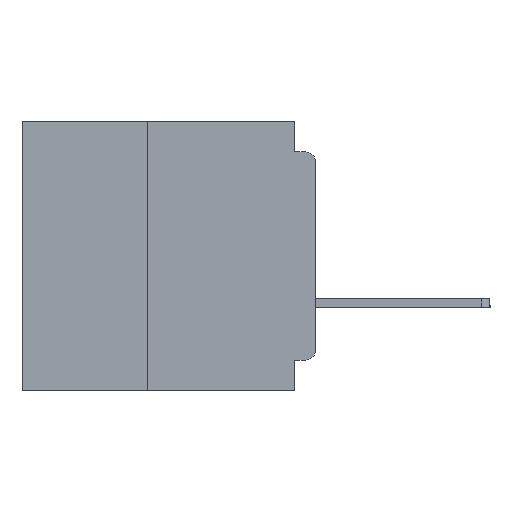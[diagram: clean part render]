
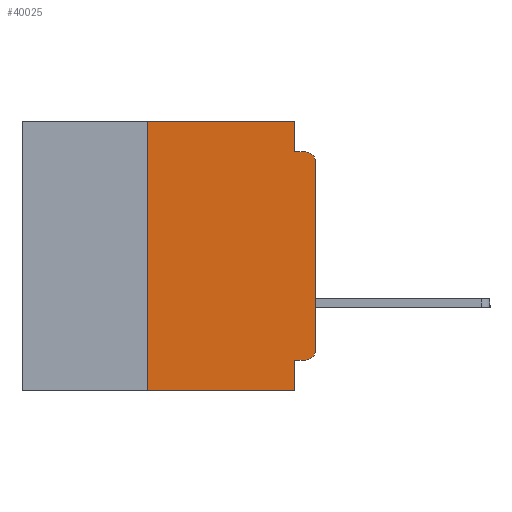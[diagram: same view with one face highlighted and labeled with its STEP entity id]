
A CAD part, left-side view. The second image highlights one B-rep face of the part: STEP entity #40025.
In plain terms, the highlighted planar face has unit normal (-1, 0, 0).
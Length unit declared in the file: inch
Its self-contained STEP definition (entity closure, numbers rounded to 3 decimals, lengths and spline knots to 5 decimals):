
#486 = LINE ( 'NONE', #40335, #39804 ) ;
#508 = VERTEX_POINT ( 'NONE', #45485 ) ;
#637 = LINE ( 'NONE', #27863, #26991 ) ;
#2961 = LINE ( 'NONE', #26568, #41119 ) ;
#3345 = LINE ( 'NONE', #22863, #11798 ) ;
#3546 = VERTEX_POINT ( 'NONE', #5297 ) ;
#5059 = CARTESIAN_POINT ( 'NONE',  ( 0., 0.031, -0.4 ) ) ;
#5124 = DIRECTION ( 'NONE',  ( 0., 1., 0. ) ) ;
#5297 = CARTESIAN_POINT ( 'NONE',  ( 0., 0.25, -0.4 ) ) ;
#5429 = DIRECTION ( 'NONE',  ( 0., 0., 1. ) ) ;
#5456 = CARTESIAN_POINT ( 'NONE',  ( 0., 0., -0.34 ) ) ;
#5501 = CARTESIAN_POINT ( 'NONE',  ( 0., 0.031, -0.4 ) ) ;
#5976 = VERTEX_POINT ( 'NONE', #9801 ) ;
#6390 = VERTEX_POINT ( 'NONE', #5501 ) ;
#8047 = VECTOR ( 'NONE', #38232, 39.37008 ) ;
#8141 = AXIS2_PLACEMENT_3D ( 'NONE', #34660, #13197, #38264 ) ;
#8829 = CARTESIAN_POINT ( 'NONE',  ( 0., 0.031, -0.045 ) ) ;
#8914 = CARTESIAN_POINT ( 'NONE',  ( 0., 0.25, -0.4 ) ) ;
#9580 = ORIENTED_EDGE ( 'NONE', *, *, #44940, .F. ) ;
#9801 = CARTESIAN_POINT ( 'NONE',  ( 0., 0., -0.06 ) ) ;
#10023 = DIRECTION ( 'NONE',  ( 0., -1., 0. ) ) ;
#10333 = LINE ( 'NONE', #45315, #29391 ) ;
#10429 = VERTEX_POINT ( 'NONE', #28794 ) ;
#10706 = CARTESIAN_POINT ( 'NONE',  ( 0., 0.031, 0. ) ) ;
#11145 = VERTEX_POINT ( 'NONE', #8829 ) ;
#11545 = VECTOR ( 'NONE', #13118, 39.37008 ) ;
#11798 = VECTOR ( 'NONE', #15829, 39.37008 ) ;
#11986 = EDGE_CURVE ( 'NONE', #11145, #28290, #637, .T. ) ;
#12305 = CARTESIAN_POINT ( 'NONE',  ( 0., 0.015, -0.045 ) ) ;
#12676 = AXIS2_PLACEMENT_3D ( 'NONE', #15783, #40872, #19360 ) ;
#12699 = CARTESIAN_POINT ( 'NONE',  ( 0., 0.015, -0.34 ) ) ;
#13118 = DIRECTION ( 'NONE',  ( 0., -1., 0. ) ) ;
#13197 = DIRECTION ( 'NONE',  ( -1., 0., 0. ) ) ;
#13347 = EDGE_CURVE ( 'NONE', #3546, #16518, #44790, .T. ) ;
#15104 = AXIS2_PLACEMENT_3D ( 'NONE', #12699, #37753, #16278 ) ;
#15783 = CARTESIAN_POINT ( 'NONE',  ( 0., 0.437, 0. ) ) ;
#15829 = DIRECTION ( 'NONE',  ( 0., -1., 0. ) ) ;
#16278 = DIRECTION ( 'NONE',  ( 0., 0., -1. ) ) ;
#16390 = ORIENTED_EDGE ( 'NONE', *, *, #33345, .F. ) ;
#16518 = VERTEX_POINT ( 'NONE', #22843 ) ;
#17746 = ORIENTED_EDGE ( 'NONE', *, *, #23326, .T. ) ;
#18140 = EDGE_CURVE ( 'NONE', #44051, #11145, #10333, .T. ) ;
#18686 = FACE_OUTER_BOUND ( 'NONE', #34059, .T. ) ;
#19211 = PLANE ( 'NONE',  #12676 ) ;
#19360 = DIRECTION ( 'NONE',  ( 0., 0., -1. ) ) ;
#21304 = EDGE_CURVE ( 'NONE', #25971, #5976, #486, .T. ) ;
#21317 = ORIENTED_EDGE ( 'NONE', *, *, #13347, .F. ) ;
#22547 = ORIENTED_EDGE ( 'NONE', *, *, #40676, .F. ) ;
#22843 = CARTESIAN_POINT ( 'NONE',  ( 0., 0.25, 0. ) ) ;
#22863 = CARTESIAN_POINT ( 'NONE',  ( 0., 0.437, 0. ) ) ;
#23326 = EDGE_CURVE ( 'NONE', #5976, #28290, #36788, .T. ) ;
#24198 = EDGE_CURVE ( 'NONE', #10429, #25971, #45353, .T. ) ;
#24756 = ORIENTED_EDGE ( 'NONE', *, *, #11986, .F. ) ;
#25653 = ORIENTED_EDGE ( 'NONE', *, *, #21304, .T. ) ;
#25971 = VERTEX_POINT ( 'NONE', #5456 ) ;
#26568 = CARTESIAN_POINT ( 'NONE',  ( 0., 0., -0.355 ) ) ;
#26991 = VECTOR ( 'NONE', #10023, 39.37008 ) ;
#27077 = LINE ( 'NONE', #5059, #8047 ) ;
#27863 = CARTESIAN_POINT ( 'NONE',  ( 0., 0., -0.045 ) ) ;
#28290 = VERTEX_POINT ( 'NONE', #12305 ) ;
#28794 = CARTESIAN_POINT ( 'NONE',  ( 0., 0.015, -0.355 ) ) ;
#29391 = VECTOR ( 'NONE', #41595, 39.37008 ) ;
#30728 = ORIENTED_EDGE ( 'NONE', *, *, #24198, .T. ) ;
#30985 = CARTESIAN_POINT ( 'NONE',  ( 0., 0.437, -0.4 ) ) ;
#32959 = ORIENTED_EDGE ( 'NONE', *, *, #18140, .F. ) ;
#33137 = DIRECTION ( 'NONE',  ( 0., 0., 1. ) ) ;
#33345 = EDGE_CURVE ( 'NONE', #16518, #44051, #3345, .T. ) ;
#34059 = EDGE_LOOP ( 'NONE', ( #25653, #17746, #24756, #32959, #16390, #21317, #45240, #22547, #9580, #30728 ) ) ;
#34660 = CARTESIAN_POINT ( 'NONE',  ( 0., 0.015, -0.06 ) ) ;
#36450 = VECTOR ( 'NONE', #5429, 39.37008 ) ;
#36788 = CIRCLE ( 'NONE', #8141, 0.015 ) ;
#37753 = DIRECTION ( 'NONE',  ( -1., 0., 0. ) ) ;
#38232 = DIRECTION ( 'NONE',  ( 0., 0., -1. ) ) ;
#38264 = DIRECTION ( 'NONE',  ( 0., 0., -1. ) ) ;
#39804 = VECTOR ( 'NONE', #33137, 39.37008 ) ;
#40025 = ADVANCED_FACE ( 'NONE', ( #18686 ), #19211, .F. ) ;
#40136 = LINE ( 'NONE', #30985, #11545 ) ;
#40335 = CARTESIAN_POINT ( 'NONE',  ( 0., 0., 0. ) ) ;
#40676 = EDGE_CURVE ( 'NONE', #508, #6390, #27077, .T. ) ;
#40872 = DIRECTION ( 'NONE',  ( 1., 0., 0. ) ) ;
#41119 = VECTOR ( 'NONE', #5124, 39.37008 ) ;
#41595 = DIRECTION ( 'NONE',  ( 0., 0., -1. ) ) ;
#43060 = EDGE_CURVE ( 'NONE', #3546, #6390, #40136, .T. ) ;
#44051 = VERTEX_POINT ( 'NONE', #10706 ) ;
#44790 = LINE ( 'NONE', #8914, #36450 ) ;
#44940 = EDGE_CURVE ( 'NONE', #10429, #508, #2961, .T. ) ;
#45240 = ORIENTED_EDGE ( 'NONE', *, *, #43060, .T. ) ;
#45315 = CARTESIAN_POINT ( 'NONE',  ( 0., 0.031, 0. ) ) ;
#45353 = CIRCLE ( 'NONE', #15104, 0.015 ) ;
#45485 = CARTESIAN_POINT ( 'NONE',  ( 0., 0.031, -0.355 ) ) ;
